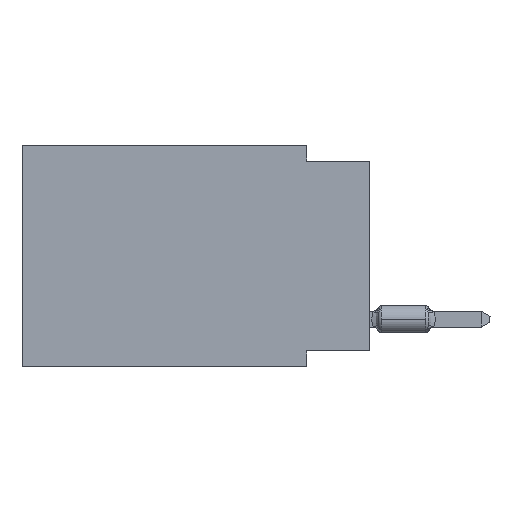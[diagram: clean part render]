
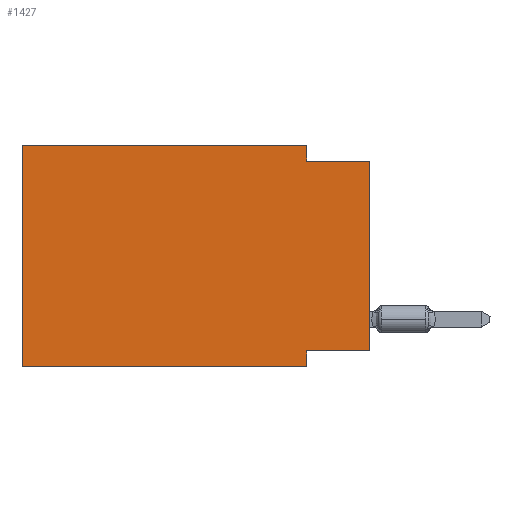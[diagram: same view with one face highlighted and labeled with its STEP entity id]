
A CAD part, left-side view. The second image highlights one B-rep face of the part: STEP entity #1427.
In plain terms, the highlighted planar face has unit normal (-1, 0, 0).
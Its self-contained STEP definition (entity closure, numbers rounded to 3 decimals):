
#147 = DIRECTION ( 'NONE',  ( 1., 0., 0. ) ) ;
#247 = VECTOR ( 'NONE', #40788, 1000. ) ;
#1427 = ADVANCED_FACE ( 'NONE', ( #24942 ), #17355, .F. ) ;
#2831 = VERTEX_POINT ( 'NONE', #52387 ) ;
#3430 = CARTESIAN_POINT ( 'NONE',  ( 0., 2.54, -8.89 ) ) ;
#4096 = DIRECTION ( 'NONE',  ( 0., 0., -1. ) ) ;
#6233 = EDGE_CURVE ( 'NONE', #22482, #37743, #54299, .T. ) ;
#8015 = VECTOR ( 'NONE', #15747, 1000. ) ;
#8592 = CARTESIAN_POINT ( 'NONE',  ( 0., 13.97, 0. ) ) ;
#8971 = ORIENTED_EDGE ( 'NONE', *, *, #9415, .F. ) ;
#9415 = EDGE_CURVE ( 'NONE', #26985, #15219, #28557, .T. ) ;
#9539 = VECTOR ( 'NONE', #24409, 1000. ) ;
#10149 = ORIENTED_EDGE ( 'NONE', *, *, #47129, .F. ) ;
#10293 = EDGE_LOOP ( 'NONE', ( #28706, #25502, #8971, #28222, #41827, #28030, #55188, #10149 ) ) ;
#11224 = EDGE_CURVE ( 'NONE', #15219, #30957, #34984, .T. ) ;
#11951 = DIRECTION ( 'NONE',  ( 0., 0., -1. ) ) ;
#13377 = CARTESIAN_POINT ( 'NONE',  ( 0., 13.97, -8.89 ) ) ;
#13651 = LINE ( 'NONE', #13377, #30897 ) ;
#15033 = CARTESIAN_POINT ( 'NONE',  ( 0., 2.54, -8.255 ) ) ;
#15219 = VERTEX_POINT ( 'NONE', #19311 ) ;
#15481 = VECTOR ( 'NONE', #11951, 1000. ) ;
#15747 = DIRECTION ( 'NONE',  ( 0., 0., 1. ) ) ;
#16716 = EDGE_CURVE ( 'NONE', #22482, #2831, #13651, .T. ) ;
#16750 = CARTESIAN_POINT ( 'NONE',  ( 0., 0., -8.255 ) ) ;
#17355 = PLANE ( 'NONE',  #36909 ) ;
#17558 = VECTOR ( 'NONE', #19203, 1000. ) ;
#17631 = CARTESIAN_POINT ( 'NONE',  ( 0., 13.97, 0. ) ) ;
#19203 = DIRECTION ( 'NONE',  ( 0., -1., 0. ) ) ;
#19311 = CARTESIAN_POINT ( 'NONE',  ( 0., 2.54, -0.635 ) ) ;
#22482 = VERTEX_POINT ( 'NONE', #35311 ) ;
#22826 = CARTESIAN_POINT ( 'NONE',  ( 0., 0., 0. ) ) ;
#24409 = DIRECTION ( 'NONE',  ( 0., 1., 0. ) ) ;
#24619 = EDGE_CURVE ( 'NONE', #26377, #30957, #53473, .T. ) ;
#24942 = FACE_OUTER_BOUND ( 'NONE', #10293, .T. ) ;
#25502 = ORIENTED_EDGE ( 'NONE', *, *, #11224, .F. ) ;
#26377 = VERTEX_POINT ( 'NONE', #16750 ) ;
#26985 = VERTEX_POINT ( 'NONE', #32581 ) ;
#28030 = ORIENTED_EDGE ( 'NONE', *, *, #16716, .T. ) ;
#28222 = ORIENTED_EDGE ( 'NONE', *, *, #46219, .F. ) ;
#28557 = LINE ( 'NONE', #33325, #15481 ) ;
#28706 = ORIENTED_EDGE ( 'NONE', *, *, #24619, .T. ) ;
#30897 = VECTOR ( 'NONE', #42638, 1000. ) ;
#30957 = VERTEX_POINT ( 'NONE', #37012 ) ;
#32581 = CARTESIAN_POINT ( 'NONE',  ( 0., 2.54, 0. ) ) ;
#33325 = CARTESIAN_POINT ( 'NONE',  ( 0., 2.54, 0. ) ) ;
#33537 = DIRECTION ( 'NONE',  ( 0., 0., -1. ) ) ;
#34984 = LINE ( 'NONE', #51885, #55141 ) ;
#35311 = CARTESIAN_POINT ( 'NONE',  ( 0., 13.97, -8.89 ) ) ;
#36909 = AXIS2_PLACEMENT_3D ( 'NONE', #17631, #147, #4096 ) ;
#37012 = CARTESIAN_POINT ( 'NONE',  ( 0., 0., -0.635 ) ) ;
#37743 = VERTEX_POINT ( 'NONE', #43801 ) ;
#39261 = VECTOR ( 'NONE', #33537, 1000. ) ;
#40294 = LINE ( 'NONE', #8592, #17558 ) ;
#40444 = CARTESIAN_POINT ( 'NONE',  ( 0., 0., -8.255 ) ) ;
#40756 = VERTEX_POINT ( 'NONE', #15033 ) ;
#40788 = DIRECTION ( 'NONE',  ( 0., 0., 1. ) ) ;
#41827 = ORIENTED_EDGE ( 'NONE', *, *, #6233, .F. ) ;
#41982 = LINE ( 'NONE', #3430, #39261 ) ;
#42638 = DIRECTION ( 'NONE',  ( 0., -1., 0. ) ) ;
#43801 = CARTESIAN_POINT ( 'NONE',  ( 0., 13.97, 0. ) ) ;
#44956 = LINE ( 'NONE', #40444, #9539 ) ;
#46219 = EDGE_CURVE ( 'NONE', #37743, #26985, #40294, .T. ) ;
#47129 = EDGE_CURVE ( 'NONE', #26377, #40756, #44956, .T. ) ;
#47669 = DIRECTION ( 'NONE',  ( 0., -1., 0. ) ) ;
#50771 = EDGE_CURVE ( 'NONE', #40756, #2831, #41982, .T. ) ;
#51885 = CARTESIAN_POINT ( 'NONE',  ( 0., 0., -0.635 ) ) ;
#52387 = CARTESIAN_POINT ( 'NONE',  ( 0., 2.54, -8.89 ) ) ;
#53473 = LINE ( 'NONE', #22826, #247 ) ;
#54299 = LINE ( 'NONE', #54855, #8015 ) ;
#54855 = CARTESIAN_POINT ( 'NONE',  ( 0., 13.97, 0. ) ) ;
#55141 = VECTOR ( 'NONE', #47669, 1000. ) ;
#55188 = ORIENTED_EDGE ( 'NONE', *, *, #50771, .F. ) ;
